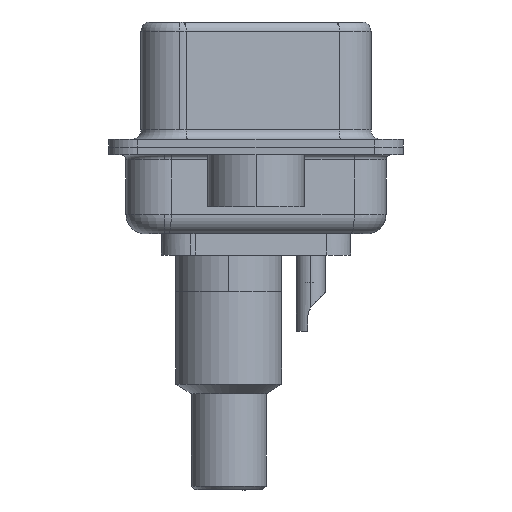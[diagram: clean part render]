
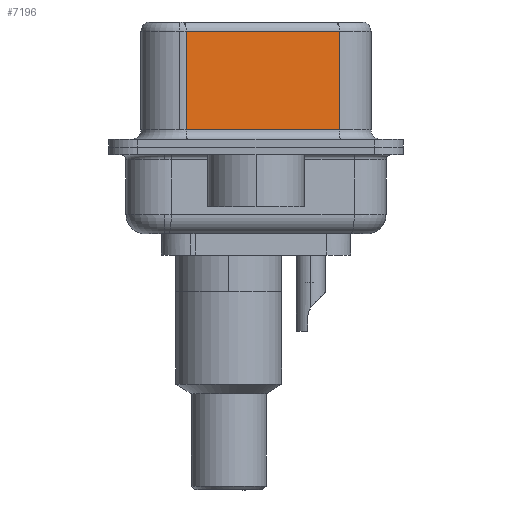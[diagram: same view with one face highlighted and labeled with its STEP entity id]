
A CAD part, left-side view. The second image highlights one B-rep face of the part: STEP entity #7196.
In plain terms, the highlighted planar face has unit normal (-0.985, -0.174, 0).
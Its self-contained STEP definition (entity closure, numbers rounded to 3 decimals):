
#258 = VECTOR ( 'NONE', #28052, 1000. ) ;
#1843 = DIRECTION ( 'NONE',  ( 0.985, 0.174, 0. ) ) ;
#1947 = EDGE_CURVE ( 'NONE', #25240, #24782, #14818, .T. ) ;
#1961 = CARTESIAN_POINT ( 'NONE',  ( 5.132, -4.322, 0.9 ) ) ;
#2691 = FACE_OUTER_BOUND ( 'NONE', #12901, .T. ) ;
#5023 = CARTESIAN_POINT ( 'NONE',  ( 5.132, -4.322, 6.02 ) ) ;
#6171 = PLANE ( 'NONE',  #18828 ) ;
#6450 = DIRECTION ( 'NONE',  ( -0.174, 0.985, 0. ) ) ;
#6692 = CARTESIAN_POINT ( 'NONE',  ( 3.73, 3.628, 6.02 ) ) ;
#6699 = ORIENTED_EDGE ( 'NONE', *, *, #1947, .T. ) ;
#7196 = ADVANCED_FACE ( 'NONE', ( #2691 ), #6171, .F. ) ;
#7467 = ORIENTED_EDGE ( 'NONE', *, *, #22523, .T. ) ;
#7766 = LINE ( 'NONE', #9168, #25384 ) ;
#7928 = DIRECTION ( 'NONE',  ( 0., 0., -1. ) ) ;
#9168 = CARTESIAN_POINT ( 'NONE',  ( 5.132, -4.322, 6.02 ) ) ;
#9849 = LINE ( 'NONE', #19342, #10192 ) ;
#10192 = VECTOR ( 'NONE', #7928, 1000. ) ;
#10530 = ORIENTED_EDGE ( 'NONE', *, *, #25050, .F. ) ;
#12277 = DIRECTION ( 'NONE',  ( 0., 0., -1. ) ) ;
#12630 = VECTOR ( 'NONE', #12277, 1000. ) ;
#12901 = EDGE_LOOP ( 'NONE', ( #10530, #14606, #6699, #7467 ) ) ;
#14606 = ORIENTED_EDGE ( 'NONE', *, *, #21465, .T. ) ;
#14818 = LINE ( 'NONE', #19072, #12630 ) ;
#17843 = DIRECTION ( 'NONE',  ( -0.174, 0.985, 0. ) ) ;
#18828 = AXIS2_PLACEMENT_3D ( 'NONE', #24756, #1843, #6450 ) ;
#18835 = CARTESIAN_POINT ( 'NONE',  ( 3.73, 3.628, 0.9 ) ) ;
#19072 = CARTESIAN_POINT ( 'NONE',  ( 3.73, 3.628, 6.52 ) ) ;
#19342 = CARTESIAN_POINT ( 'NONE',  ( 5.132, -4.322, 6.52 ) ) ;
#20759 = VERTEX_POINT ( 'NONE', #1961 ) ;
#21465 = EDGE_CURVE ( 'NONE', #25682, #25240, #7766, .T. ) ;
#22523 = EDGE_CURVE ( 'NONE', #24782, #20759, #22577, .T. ) ;
#22577 = LINE ( 'NONE', #23669, #258 ) ;
#23669 = CARTESIAN_POINT ( 'NONE',  ( 5.132, -4.322, 0.9 ) ) ;
#24756 = CARTESIAN_POINT ( 'NONE',  ( 5.132, -4.322, 6.52 ) ) ;
#24782 = VERTEX_POINT ( 'NONE', #18835 ) ;
#25050 = EDGE_CURVE ( 'NONE', #25682, #20759, #9849, .T. ) ;
#25240 = VERTEX_POINT ( 'NONE', #6692 ) ;
#25384 = VECTOR ( 'NONE', #17843, 1000. ) ;
#25682 = VERTEX_POINT ( 'NONE', #5023 ) ;
#28052 = DIRECTION ( 'NONE',  ( 0.174, -0.985, 0. ) ) ;
